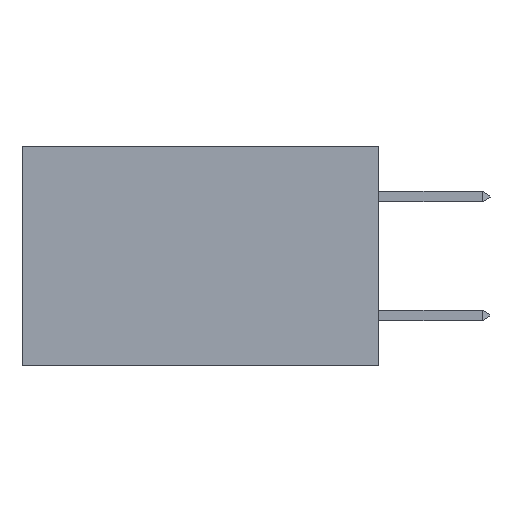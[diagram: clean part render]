
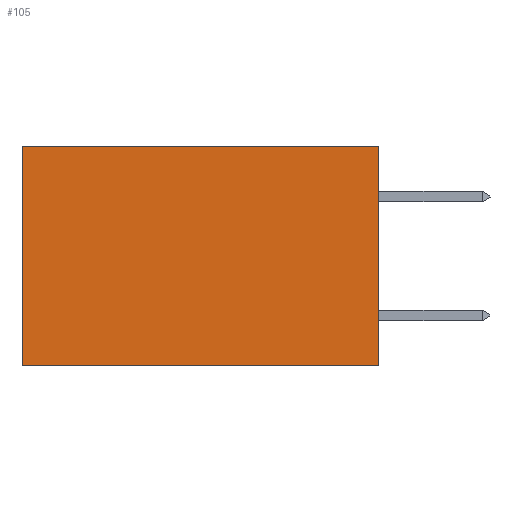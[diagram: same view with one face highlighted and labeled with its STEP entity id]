
A CAD part, left-side view. The second image highlights one B-rep face of the part: STEP entity #105.
In plain terms, the highlighted planar face has unit normal (-1, 0, 0).
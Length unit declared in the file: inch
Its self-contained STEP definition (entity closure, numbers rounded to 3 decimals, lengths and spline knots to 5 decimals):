
#105 = ADVANCED_FACE ( 'NONE', ( #7051 ), #6385, .F. ) ;
#412 = EDGE_CURVE ( 'NONE', #18478, #4827, #21219, .T. ) ;
#447 = EDGE_CURVE ( 'NONE', #18478, #2967, #15049, .T. ) ;
#2140 = ORIENTED_EDGE ( 'NONE', *, *, #412, .T. ) ;
#2308 = LINE ( 'NONE', #10008, #12617 ) ;
#2967 = VERTEX_POINT ( 'NONE', #6392 ) ;
#4124 = VECTOR ( 'NONE', #4142, 39.37008 ) ;
#4142 = DIRECTION ( 'NONE',  ( 0., 0., -1. ) ) ;
#4827 = VERTEX_POINT ( 'NONE', #18246 ) ;
#4860 = ORIENTED_EDGE ( 'NONE', *, *, #7956, .T. ) ;
#6307 = CARTESIAN_POINT ( 'NONE',  ( 0.298, 0.6, -0.37 ) ) ;
#6385 = PLANE ( 'NONE',  #10283 ) ;
#6392 = CARTESIAN_POINT ( 'NONE',  ( 0.298, 0., -0.37 ) ) ;
#7051 = FACE_OUTER_BOUND ( 'NONE', #14049, .T. ) ;
#7956 = EDGE_CURVE ( 'NONE', #4827, #8509, #21124, .T. ) ;
#8220 = DIRECTION ( 'NONE',  ( 0., 0., -1. ) ) ;
#8509 = VERTEX_POINT ( 'NONE', #6307 ) ;
#10008 = CARTESIAN_POINT ( 'NONE',  ( 0.298, 0., -0.37 ) ) ;
#10146 = CARTESIAN_POINT ( 'NONE',  ( 0.298, 0., 0. ) ) ;
#10182 = ORIENTED_EDGE ( 'NONE', *, *, #12671, .F. ) ;
#10283 = AXIS2_PLACEMENT_3D ( 'NONE', #23583, #18991, #8220 ) ;
#10868 = VECTOR ( 'NONE', #11790, 39.37008 ) ;
#11790 = DIRECTION ( 'NONE',  ( 0., 1., 0. ) ) ;
#12095 = DIRECTION ( 'NONE',  ( 0., 1., 0. ) ) ;
#12617 = VECTOR ( 'NONE', #12095, 39.37008 ) ;
#12671 = EDGE_CURVE ( 'NONE', #2967, #8509, #2308, .T. ) ;
#12679 = CARTESIAN_POINT ( 'NONE',  ( 0.298, 0., 0. ) ) ;
#14049 = EDGE_LOOP ( 'NONE', ( #4860, #10182, #16848, #2140 ) ) ;
#14096 = CARTESIAN_POINT ( 'NONE',  ( 0.298, 0., 0. ) ) ;
#14455 = DIRECTION ( 'NONE',  ( 0., 0., -1. ) ) ;
#15049 = LINE ( 'NONE', #10146, #4124 ) ;
#16848 = ORIENTED_EDGE ( 'NONE', *, *, #447, .F. ) ;
#18246 = CARTESIAN_POINT ( 'NONE',  ( 0.298, 0.6, 0. ) ) ;
#18478 = VERTEX_POINT ( 'NONE', #12679 ) ;
#18991 = DIRECTION ( 'NONE',  ( 1., 0., 0. ) ) ;
#21124 = LINE ( 'NONE', #24751, #24638 ) ;
#21219 = LINE ( 'NONE', #14096, #10868 ) ;
#23583 = CARTESIAN_POINT ( 'NONE',  ( 0.298, 0., 0. ) ) ;
#24638 = VECTOR ( 'NONE', #14455, 39.37008 ) ;
#24751 = CARTESIAN_POINT ( 'NONE',  ( 0.298, 0.6, 0. ) ) ;
